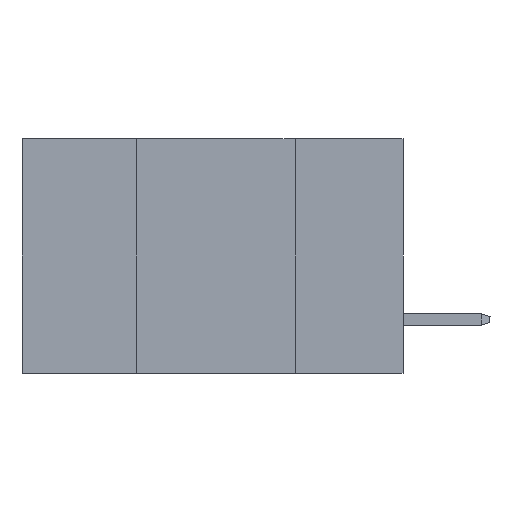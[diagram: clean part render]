
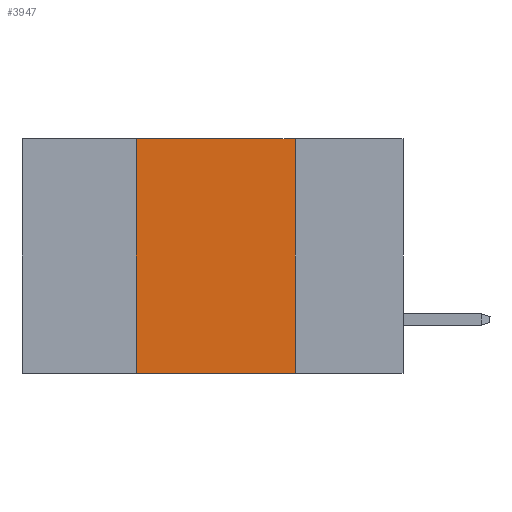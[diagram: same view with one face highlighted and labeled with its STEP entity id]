
A CAD part, left-side view. The second image highlights one B-rep face of the part: STEP entity #3947.
In plain terms, the highlighted planar face has unit normal (-1, 0, 0).
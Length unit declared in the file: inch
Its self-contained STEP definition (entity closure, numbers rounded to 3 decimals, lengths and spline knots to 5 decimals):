
#1986 = CARTESIAN_POINT ( 'NONE',  ( 0., 0.17, 0. ) ) ;
#3497 = DIRECTION ( 'NONE',  ( 0., 0., -1. ) ) ;
#3764 = VECTOR ( 'NONE', #19105, 39.37008 ) ;
#3947 = ADVANCED_FACE ( 'NONE', ( #15160 ), #29392, .F. ) ;
#4259 = CARTESIAN_POINT ( 'NONE',  ( 0., 0.42, 0. ) ) ;
#4704 = VERTEX_POINT ( 'NONE', #16861 ) ;
#5339 = CARTESIAN_POINT ( 'NONE',  ( 0., 0.6, 0. ) ) ;
#5468 = VERTEX_POINT ( 'NONE', #4259 ) ;
#5638 = VECTOR ( 'NONE', #22389, 39.37008 ) ;
#6077 = ORIENTED_EDGE ( 'NONE', *, *, #27086, .F. ) ;
#7608 = ORIENTED_EDGE ( 'NONE', *, *, #14898, .T. ) ;
#8342 = LINE ( 'NONE', #24670, #26745 ) ;
#8467 = VECTOR ( 'NONE', #28715, 39.37008 ) ;
#8635 = LINE ( 'NONE', #20287, #5638 ) ;
#9476 = VERTEX_POINT ( 'NONE', #1986 ) ;
#9892 = LINE ( 'NONE', #5339, #3764 ) ;
#10282 = CARTESIAN_POINT ( 'NONE',  ( 0., 0.6, -0.37 ) ) ;
#11281 = AXIS2_PLACEMENT_3D ( 'NONE', #24087, #28778, #3497 ) ;
#12249 = LINE ( 'NONE', #10282, #8467 ) ;
#13637 = ORIENTED_EDGE ( 'NONE', *, *, #18662, .F. ) ;
#14622 = ORIENTED_EDGE ( 'NONE', *, *, #16363, .F. ) ;
#14898 = EDGE_CURVE ( 'NONE', #4704, #21278, #12249, .T. ) ;
#15160 = FACE_OUTER_BOUND ( 'NONE', #18275, .T. ) ;
#16363 = EDGE_CURVE ( 'NONE', #4704, #5468, #8635, .T. ) ;
#16861 = CARTESIAN_POINT ( 'NONE',  ( 0., 0.42, -0.37 ) ) ;
#17575 = DIRECTION ( 'NONE',  ( 0., 0., -1. ) ) ;
#18275 = EDGE_LOOP ( 'NONE', ( #13637, #6077, #14622, #7608 ) ) ;
#18662 = EDGE_CURVE ( 'NONE', #9476, #21278, #8342, .T. ) ;
#19105 = DIRECTION ( 'NONE',  ( 0., -1., 0. ) ) ;
#20287 = CARTESIAN_POINT ( 'NONE',  ( 0., 0.42, 0. ) ) ;
#21278 = VERTEX_POINT ( 'NONE', #27256 ) ;
#22389 = DIRECTION ( 'NONE',  ( 0., 0., 1. ) ) ;
#24087 = CARTESIAN_POINT ( 'NONE',  ( 0., 0.6, 0. ) ) ;
#24670 = CARTESIAN_POINT ( 'NONE',  ( 0., 0.17, 0. ) ) ;
#26745 = VECTOR ( 'NONE', #17575, 39.37008 ) ;
#27086 = EDGE_CURVE ( 'NONE', #5468, #9476, #9892, .T. ) ;
#27256 = CARTESIAN_POINT ( 'NONE',  ( 0., 0.17, -0.37 ) ) ;
#28715 = DIRECTION ( 'NONE',  ( 0., -1., 0. ) ) ;
#28778 = DIRECTION ( 'NONE',  ( 1., 0., 0. ) ) ;
#29392 = PLANE ( 'NONE',  #11281 ) ;
